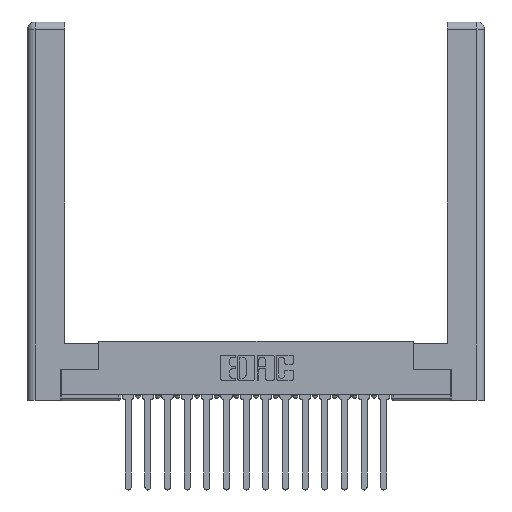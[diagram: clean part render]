
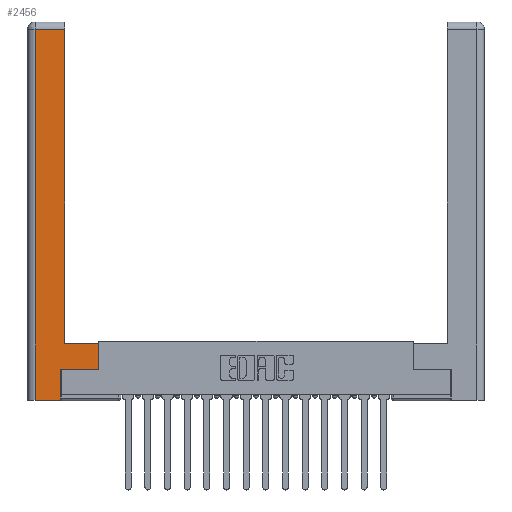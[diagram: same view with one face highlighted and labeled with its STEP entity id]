
A CAD part, top view. The second image highlights one B-rep face of the part: STEP entity #2456.
In plain terms, the highlighted planar face has unit normal (0, 0, 1).
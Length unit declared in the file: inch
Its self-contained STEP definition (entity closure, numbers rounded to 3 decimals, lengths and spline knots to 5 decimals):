
#20 = LINE ( 'NONE', #12641, #565 ) ;
#327 = DIRECTION ( 'NONE',  ( 1., 0., 0. ) ) ;
#433 = DIRECTION ( 'NONE',  ( -1., 0., 0. ) ) ;
#565 = VECTOR ( 'NONE', #17942, 39.37008 ) ;
#1135 = CARTESIAN_POINT ( 'NONE',  ( 0., 0., 0. ) ) ;
#1412 = CARTESIAN_POINT ( 'NONE',  ( 0.565, 0.45, 0. ) ) ;
#1535 = CARTESIAN_POINT ( 'NONE',  ( 0.0615, 2.94, 0. ) ) ;
#1643 = CARTESIAN_POINT ( 'NONE',  ( 0.0615, 0., 0. ) ) ;
#1867 = VECTOR ( 'NONE', #10897, 39.37008 ) ;
#2026 = EDGE_CURVE ( 'NONE', #16022, #4545, #8819, .T. ) ;
#2220 = VERTEX_POINT ( 'NONE', #16686 ) ;
#2456 = ADVANCED_FACE ( 'NONE', ( #13576 ), #12206, .F. ) ;
#2491 = LINE ( 'NONE', #8053, #1867 ) ;
#2513 = VECTOR ( 'NONE', #433, 39.37008 ) ;
#3113 = CARTESIAN_POINT ( 'NONE',  ( 0.265, 0., 0. ) ) ;
#3152 = LINE ( 'NONE', #14833, #11519 ) ;
#3664 = VERTEX_POINT ( 'NONE', #1535 ) ;
#3678 = DIRECTION ( 'NONE',  ( 0., -1., 0. ) ) ;
#4220 = CARTESIAN_POINT ( 'NONE',  ( 0.295, 2.94, 0. ) ) ;
#4276 = VERTEX_POINT ( 'NONE', #12628 ) ;
#4545 = VERTEX_POINT ( 'NONE', #3113 ) ;
#5764 = LINE ( 'NONE', #11335, #2513 ) ;
#6238 = CARTESIAN_POINT ( 'NONE',  ( 0.265, 0.245, 0. ) ) ;
#6851 = EDGE_CURVE ( 'NONE', #14768, #14301, #17758, .T. ) ;
#6887 = EDGE_CURVE ( 'NONE', #14301, #3664, #20, .T. ) ;
#6972 = VECTOR ( 'NONE', #14196, 39.37008 ) ;
#7333 = VERTEX_POINT ( 'NONE', #1412 ) ;
#7504 = ORIENTED_EDGE ( 'NONE', *, *, #12126, .T. ) ;
#8053 = CARTESIAN_POINT ( 'NONE',  ( 0.565, 0.45, 0. ) ) ;
#8278 = ORIENTED_EDGE ( 'NONE', *, *, #6887, .T. ) ;
#8819 = LINE ( 'NONE', #10371, #16843 ) ;
#9016 = ORIENTED_EDGE ( 'NONE', *, *, #17509, .T. ) ;
#9048 = DIRECTION ( 'NONE',  ( 0., 1., 0. ) ) ;
#9075 = DIRECTION ( 'NONE',  ( 0., 0., -1. ) ) ;
#9167 = VECTOR ( 'NONE', #13876, 39.37008 ) ;
#9739 = LINE ( 'NONE', #16862, #9167 ) ;
#10160 = VECTOR ( 'NONE', #9048, 39.37008 ) ;
#10371 = CARTESIAN_POINT ( 'NONE',  ( 0.265, 0., 0. ) ) ;
#10822 = DIRECTION ( 'NONE',  ( -1., 0., 0. ) ) ;
#10897 = DIRECTION ( 'NONE',  ( 0., 1., 0. ) ) ;
#11043 = EDGE_CURVE ( 'NONE', #2220, #7333, #2491, .T. ) ;
#11335 = CARTESIAN_POINT ( 'NONE',  ( 0.295, 0.45, 0. ) ) ;
#11519 = VECTOR ( 'NONE', #3678, 39.37008 ) ;
#11763 = ORIENTED_EDGE ( 'NONE', *, *, #6851, .T. ) ;
#11958 = EDGE_CURVE ( 'NONE', #4276, #2220, #9739, .T. ) ;
#12126 = EDGE_CURVE ( 'NONE', #3664, #16022, #3152, .T. ) ;
#12206 = PLANE ( 'NONE',  #17225 ) ;
#12272 = ORIENTED_EDGE ( 'NONE', *, *, #14762, .T. ) ;
#12628 = CARTESIAN_POINT ( 'NONE',  ( 0.265, 0.245, 0. ) ) ;
#12641 = CARTESIAN_POINT ( 'NONE',  ( 0.0615, 2.94, 0. ) ) ;
#12895 = EDGE_LOOP ( 'NONE', ( #11763, #8278, #7504, #15826, #9016, #18040, #17136, #12272 ) ) ;
#13576 = FACE_OUTER_BOUND ( 'NONE', #12895, .T. ) ;
#13660 = CARTESIAN_POINT ( 'NONE',  ( 0.295, 3., 0. ) ) ;
#13876 = DIRECTION ( 'NONE',  ( 1., 0., 0. ) ) ;
#14196 = DIRECTION ( 'NONE',  ( 0., 1., 0. ) ) ;
#14301 = VERTEX_POINT ( 'NONE', #4220 ) ;
#14762 = EDGE_CURVE ( 'NONE', #7333, #14768, #5764, .T. ) ;
#14768 = VERTEX_POINT ( 'NONE', #16893 ) ;
#14833 = CARTESIAN_POINT ( 'NONE',  ( 0.0615, 0., 0. ) ) ;
#15826 = ORIENTED_EDGE ( 'NONE', *, *, #2026, .T. ) ;
#16022 = VERTEX_POINT ( 'NONE', #1643 ) ;
#16686 = CARTESIAN_POINT ( 'NONE',  ( 0.565, 0.245, 0. ) ) ;
#16843 = VECTOR ( 'NONE', #327, 39.37008 ) ;
#16862 = CARTESIAN_POINT ( 'NONE',  ( 0.565, 0.245, 0. ) ) ;
#16893 = CARTESIAN_POINT ( 'NONE',  ( 0.295, 0.45, 0. ) ) ;
#17136 = ORIENTED_EDGE ( 'NONE', *, *, #11043, .T. ) ;
#17225 = AXIS2_PLACEMENT_3D ( 'NONE', #1135, #9075, #10822 ) ;
#17463 = LINE ( 'NONE', #6238, #10160 ) ;
#17509 = EDGE_CURVE ( 'NONE', #4545, #4276, #17463, .T. ) ;
#17758 = LINE ( 'NONE', #13660, #6972 ) ;
#17942 = DIRECTION ( 'NONE',  ( -1., 0., 0. ) ) ;
#18040 = ORIENTED_EDGE ( 'NONE', *, *, #11958, .T. ) ;
